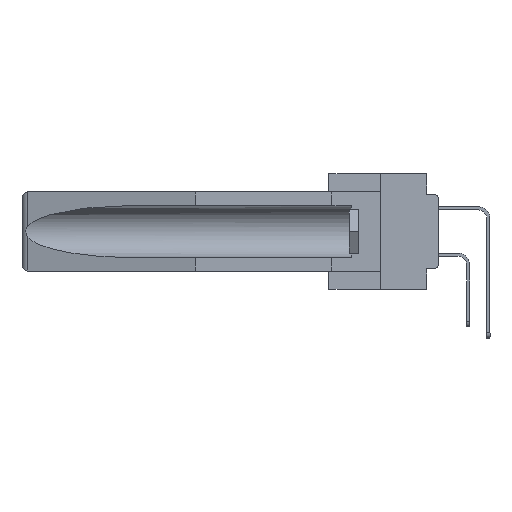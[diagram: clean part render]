
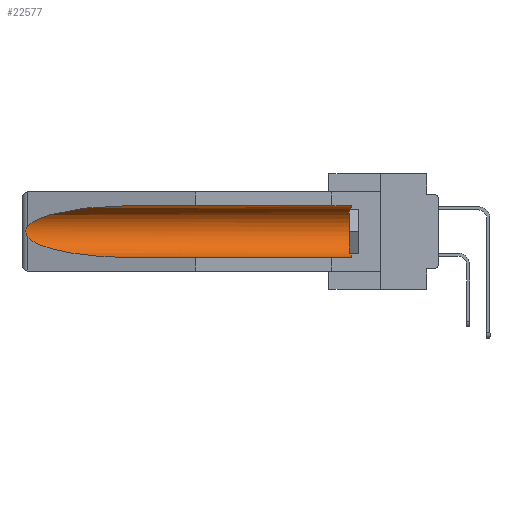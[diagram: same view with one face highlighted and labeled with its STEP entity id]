
A CAD part, left-side view. The second image highlights one B-rep face of the part: STEP entity #22577.
In plain terms, the highlighted cylindrical face has radius 2.857 mm (diameter 5.715 mm), a partial arc.
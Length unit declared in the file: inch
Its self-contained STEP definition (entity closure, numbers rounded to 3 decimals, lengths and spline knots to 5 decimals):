
#1005 = CIRCLE ( 'NONE', #12714, 0.1125 ) ;
#1262 = VECTOR ( 'NONE', #13434, 39.37008 ) ;
#1528 = CARTESIAN_POINT ( 'NONE',  ( 0.25451, 1.48313, -0.09465 ) ) ;
#1722 = CARTESIAN_POINT ( 'NONE',  ( 0.155, 1.07973, -0.059 ) ) ;
#2193 = CARTESIAN_POINT ( 'NONE',  ( 0.2673, 1.5327, -0.16383 ) ) ;
#2756 = CARTESIAN_POINT ( 'NONE',  ( 0.21114, 1.30732, -0.284 ) ) ;
#2868 = CARTESIAN_POINT ( 'NONE',  ( 0.26537, 1.52718, -0.19328 ) ) ;
#3064 = VERTEX_POINT ( 'NONE', #2868 ) ;
#3295 = DIRECTION ( 'NONE',  ( 0., 1., 0. ) ) ;
#5083 = EDGE_LOOP ( 'NONE', ( #14851, #26877, #11699, #34355, #19124, #28820 ) ) ;
#7249 = CARTESIAN_POINT ( 'NONE',  ( 0.155, 0.126, -0.284 ) ) ;
#7569 = VECTOR ( 'NONE', #37199, 39.37008 ) ;
#8517 = CYLINDRICAL_SURFACE ( 'NONE', #11777, 0.1125 ) ;
#8704 = FACE_OUTER_BOUND ( 'NONE', #5083, .T. ) ;
#9530 = CARTESIAN_POINT ( 'NONE',  ( 0.155, 1.07973, -0.284 ) ) ;
#10420 = CARTESIAN_POINT ( 'NONE',  ( 0.26537, 1.52718, -0.14972 ) ) ;
#10568 = CARTESIAN_POINT ( 'NONE',  ( 0.155, 0.126, -0.1715 ) ) ;
#10717 = EDGE_CURVE ( 'NONE', #13918, #14901, #18833, .T. ) ;
#11085 = CARTESIAN_POINT ( 'NONE',  ( 0.26537, 1.52718, -0.19328 ) ) ;
#11686 = EDGE_CURVE ( 'NONE', #27716, #18554, #22237, .T. ) ;
#11699 = ORIENTED_EDGE ( 'NONE', *, *, #29737, .T. ) ;
#11777 = AXIS2_PLACEMENT_3D ( 'NONE', #17983, #3295, #23397 ) ;
#12714 = AXIS2_PLACEMENT_3D ( 'NONE', #10568, #28523, #20030 ) ;
#13285 = CARTESIAN_POINT ( 'NONE',  ( 0.155, 0.126, -0.059 ) ) ;
#13434 = DIRECTION ( 'NONE',  ( 0., 1., 0. ) ) ;
#13500 = CARTESIAN_POINT ( 'NONE',  ( 0.21114, 1.30732, -0.059 ) ) ;
#13624 = EDGE_CURVE ( 'NONE', #13918, #15856, #1005, .T. ) ;
#13918 = VERTEX_POINT ( 'NONE', #7249 ) ;
#13973 = CARTESIAN_POINT ( 'NONE',  ( 0.2675, 1.53308, -0.17534 ) ) ;
#14851 = ORIENTED_EDGE ( 'NONE', *, *, #11686, .T. ) ;
#14901 = VERTEX_POINT ( 'NONE', #9530 ) ;
#15856 = VERTEX_POINT ( 'NONE', #13285 ) ;
#16113 = CARTESIAN_POINT ( 'NONE',  ( 0.26597, 1.5296, -0.19026 ) ) ;
#16687 = CARTESIAN_POINT ( 'NONE',  ( 0.26654, 1.53092, -0.15636 ) ) ;
#17983 = CARTESIAN_POINT ( 'NONE',  ( 0.155, -0.30754, -0.1715 ) ) ;
#18554 = VERTEX_POINT ( 'NONE', #19666 ) ;
#18833 = LINE ( 'NONE', #30621, #7569 ) ;
#19124 = ORIENTED_EDGE ( 'NONE', *, *, #13624, .T. ) ;
#19666 = CARTESIAN_POINT ( 'NONE',  ( 0.26537, 1.52718, -0.14972 ) ) ;
#19973 = CARTESIAN_POINT ( 'NONE',  ( 0.2675, 1.53308, -0.16763 ) ) ;
#20030 = DIRECTION ( 'NONE',  ( 0., 0., 1. ) ) ;
#20932 = CARTESIAN_POINT ( 'NONE',  ( 0.25451, 1.48313, -0.24835 ) ) ;
#22237 =( BOUNDED_CURVE ( )  B_SPLINE_CURVE ( 3, ( #1722, #13500, #1528, #10420 ),
 .UNSPECIFIED., .F., .T. ) 
 B_SPLINE_CURVE_WITH_KNOTS ( ( 4, 4 ),
 ( 4.71239, 6.08839 ),
 .UNSPECIFIED. ) 
 CURVE ( )  GEOMETRIC_REPRESENTATION_ITEM ( )  RATIONAL_B_SPLINE_CURVE ( ( 1., 0.848, 0.848, 1. ) ) 
 REPRESENTATION_ITEM ( '' )  );
#22577 = ADVANCED_FACE ( 'NONE', ( #8704 ), #8517, .F. ) ;
#23397 = DIRECTION ( 'NONE',  ( 0., 0., 1. ) ) ;
#23474 =( BOUNDED_CURVE ( )  B_SPLINE_CURVE ( 3, ( #35629, #20932, #2756, #35431 ),
 .UNSPECIFIED., .F., .F. ) 
 B_SPLINE_CURVE_WITH_KNOTS ( ( 4, 4 ),
 ( 0.1948, 1.5708 ),
 .UNSPECIFIED. ) 
 CURVE ( )  GEOMETRIC_REPRESENTATION_ITEM ( )  RATIONAL_B_SPLINE_CURVE ( ( 1., 0.848, 0.848, 1. ) ) 
 REPRESENTATION_ITEM ( '' )  );
#25025 = CARTESIAN_POINT ( 'NONE',  ( 0.155, -0.30754, -0.059 ) ) ;
#26877 = ORIENTED_EDGE ( 'NONE', *, *, #37142, .T. ) ;
#27174 = CARTESIAN_POINT ( 'NONE',  ( 0.155, 1.07973, -0.059 ) ) ;
#27716 = VERTEX_POINT ( 'NONE', #27174 ) ;
#28092 = CARTESIAN_POINT ( 'NONE',  ( 0.26597, 1.52961, -0.15275 ) ) ;
#28464 = CARTESIAN_POINT ( 'NONE',  ( 0.26655, 1.53094, -0.18657 ) ) ;
#28523 = DIRECTION ( 'NONE',  ( 0., -1., 0. ) ) ;
#28820 = ORIENTED_EDGE ( 'NONE', *, *, #34229, .T. ) ;
#29737 = EDGE_CURVE ( 'NONE', #3064, #14901, #23474, .T. ) ;
#30621 = CARTESIAN_POINT ( 'NONE',  ( 0.155, -0.30754, -0.284 ) ) ;
#34099 = CARTESIAN_POINT ( 'NONE',  ( 0.2673, 1.53269, -0.17917 ) ) ;
#34229 = EDGE_CURVE ( 'NONE', #15856, #27716, #37029, .T. ) ;
#34355 = ORIENTED_EDGE ( 'NONE', *, *, #10717, .F. ) ;
#35431 = CARTESIAN_POINT ( 'NONE',  ( 0.155, 1.07973, -0.284 ) ) ;
#35629 = CARTESIAN_POINT ( 'NONE',  ( 0.26537, 1.52718, -0.19328 ) ) ;
#36761 = B_SPLINE_CURVE_WITH_KNOTS ( 'NONE', 3,
 ( #37003, #28092, #16687, #2193, #19973, #13973, #34099, #28464, #16113, #11085 ),
 .UNSPECIFIED., .F., .F.,
 ( 4, 2, 2, 2, 4 ),
 ( 0., 0.00029, 0.00058, 0.00087, 0.00117 ),
 .UNSPECIFIED. ) ;
#37003 = CARTESIAN_POINT ( 'NONE',  ( 0.26537, 1.52718, -0.14972 ) ) ;
#37029 = LINE ( 'NONE', #25025, #1262 ) ;
#37142 = EDGE_CURVE ( 'NONE', #18554, #3064, #36761, .T. ) ;
#37199 = DIRECTION ( 'NONE',  ( 0., 1., 0. ) ) ;
